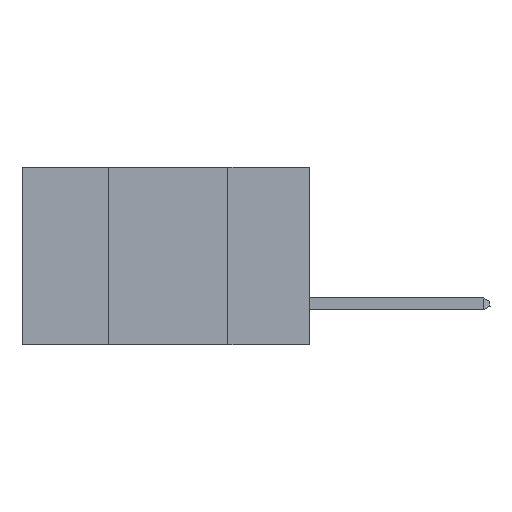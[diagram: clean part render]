
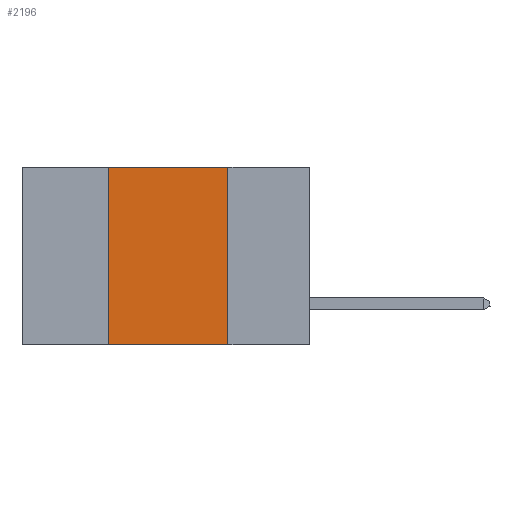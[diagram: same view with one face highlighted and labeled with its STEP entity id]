
A CAD part, left-side view. The second image highlights one B-rep face of the part: STEP entity #2196.
In plain terms, the highlighted planar face has unit normal (-1, 0, 0).
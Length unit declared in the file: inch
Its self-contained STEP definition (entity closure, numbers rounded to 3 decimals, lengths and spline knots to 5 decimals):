
#210 = CARTESIAN_POINT ( 'NONE',  ( 0., 0.17, 0. ) ) ;
#782 = DIRECTION ( 'NONE',  ( 1., 0., 0. ) ) ;
#879 = VERTEX_POINT ( 'NONE', #4478 ) ;
#1163 = FACE_OUTER_BOUND ( 'NONE', #11035, .T. ) ;
#1421 = ORIENTED_EDGE ( 'NONE', *, *, #2455, .T. ) ;
#1756 = DIRECTION ( 'NONE',  ( 0., -1., 0. ) ) ;
#1909 = CARTESIAN_POINT ( 'NONE',  ( 0., 0.17, -0.37 ) ) ;
#2196 = ADVANCED_FACE ( 'NONE', ( #1163 ), #8440, .F. ) ;
#2305 = EDGE_CURVE ( 'NONE', #879, #6701, #9889, .T. ) ;
#2455 = EDGE_CURVE ( 'NONE', #12757, #8461, #2707, .T. ) ;
#2707 = LINE ( 'NONE', #9450, #6570 ) ;
#3248 = VECTOR ( 'NONE', #1756, 39.37008 ) ;
#3919 = EDGE_CURVE ( 'NONE', #6701, #8461, #4470, .T. ) ;
#4470 = LINE ( 'NONE', #210, #12325 ) ;
#4478 = CARTESIAN_POINT ( 'NONE',  ( 0., 0.42, 0. ) ) ;
#4785 = CARTESIAN_POINT ( 'NONE',  ( 0., 0.42, -0.37 ) ) ;
#5338 = DIRECTION ( 'NONE',  ( 0., -1., 0. ) ) ;
#5598 = DIRECTION ( 'NONE',  ( 0., 0., 1. ) ) ;
#6390 = DIRECTION ( 'NONE',  ( 0., 0., -1. ) ) ;
#6428 = EDGE_CURVE ( 'NONE', #12757, #879, #9493, .T. ) ;
#6570 = VECTOR ( 'NONE', #5338, 39.37008 ) ;
#6701 = VERTEX_POINT ( 'NONE', #11557 ) ;
#6880 = CARTESIAN_POINT ( 'NONE',  ( 0., 0.42, 0. ) ) ;
#6910 = ORIENTED_EDGE ( 'NONE', *, *, #3919, .F. ) ;
#8013 = DIRECTION ( 'NONE',  ( 0., 0., -1. ) ) ;
#8440 = PLANE ( 'NONE',  #11008 ) ;
#8461 = VERTEX_POINT ( 'NONE', #1909 ) ;
#9450 = CARTESIAN_POINT ( 'NONE',  ( 0., 0.6, -0.37 ) ) ;
#9493 = LINE ( 'NONE', #6880, #11906 ) ;
#9889 = LINE ( 'NONE', #13855, #3248 ) ;
#10071 = ORIENTED_EDGE ( 'NONE', *, *, #6428, .F. ) ;
#11008 = AXIS2_PLACEMENT_3D ( 'NONE', #12872, #782, #6390 ) ;
#11035 = EDGE_LOOP ( 'NONE', ( #6910, #12889, #10071, #1421 ) ) ;
#11557 = CARTESIAN_POINT ( 'NONE',  ( 0., 0.17, 0. ) ) ;
#11906 = VECTOR ( 'NONE', #5598, 39.37008 ) ;
#12325 = VECTOR ( 'NONE', #8013, 39.37008 ) ;
#12757 = VERTEX_POINT ( 'NONE', #4785 ) ;
#12872 = CARTESIAN_POINT ( 'NONE',  ( 0., 0.6, 0. ) ) ;
#12889 = ORIENTED_EDGE ( 'NONE', *, *, #2305, .F. ) ;
#13855 = CARTESIAN_POINT ( 'NONE',  ( 0., 0.6, 0. ) ) ;
